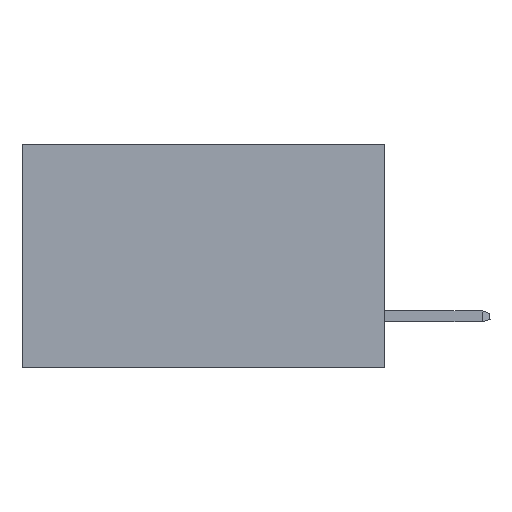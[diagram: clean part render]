
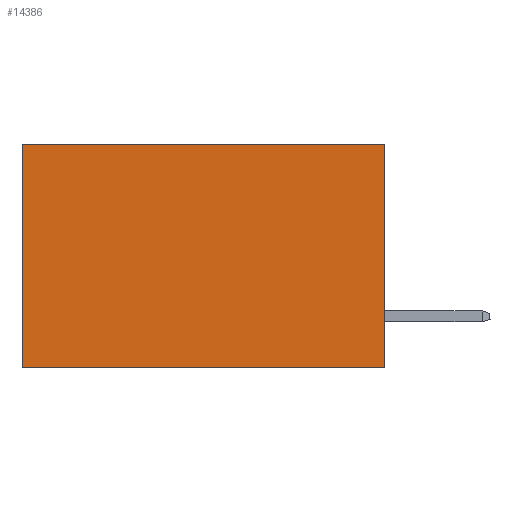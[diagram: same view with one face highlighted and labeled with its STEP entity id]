
A CAD part, left-side view. The second image highlights one B-rep face of the part: STEP entity #14386.
In plain terms, the highlighted planar face has unit normal (-1, 0, 0).
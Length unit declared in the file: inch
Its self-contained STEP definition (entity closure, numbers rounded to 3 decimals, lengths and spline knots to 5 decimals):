
#104 = VECTOR ( 'NONE', #4409, 39.37008 ) ;
#169 = VECTOR ( 'NONE', #10828, 39.37008 ) ;
#344 = ORIENTED_EDGE ( 'NONE', *, *, #9839, .F. ) ;
#633 = DIRECTION ( 'NONE',  ( 0., 0., -1. ) ) ;
#2063 = CARTESIAN_POINT ( 'NONE',  ( 0.298, 0.6, 0. ) ) ;
#2484 = ORIENTED_EDGE ( 'NONE', *, *, #14742, .T. ) ;
#2728 = ORIENTED_EDGE ( 'NONE', *, *, #3739, .F. ) ;
#3150 = CARTESIAN_POINT ( 'NONE',  ( 0.298, 0., 0. ) ) ;
#3463 = CARTESIAN_POINT ( 'NONE',  ( 0.298, 0.6, -0.37 ) ) ;
#3540 = VERTEX_POINT ( 'NONE', #12325 ) ;
#3739 = EDGE_CURVE ( 'NONE', #7100, #16364, #4299, .T. ) ;
#3740 = DIRECTION ( 'NONE',  ( 0., 1., 0. ) ) ;
#3833 = LINE ( 'NONE', #9637, #4688 ) ;
#4299 = LINE ( 'NONE', #13336, #6196 ) ;
#4409 = DIRECTION ( 'NONE',  ( 0., 1., 0. ) ) ;
#4688 = VECTOR ( 'NONE', #13706, 39.37008 ) ;
#6084 = PLANE ( 'NONE',  #12268 ) ;
#6181 = VERTEX_POINT ( 'NONE', #13823 ) ;
#6196 = VECTOR ( 'NONE', #3740, 39.37008 ) ;
#7100 = VERTEX_POINT ( 'NONE', #10840 ) ;
#7273 = LINE ( 'NONE', #3150, #104 ) ;
#8187 = LINE ( 'NONE', #2063, #169 ) ;
#8215 = EDGE_CURVE ( 'NONE', #6181, #3540, #7273, .T. ) ;
#8732 = CARTESIAN_POINT ( 'NONE',  ( 0.298, 0., 0. ) ) ;
#8881 = ORIENTED_EDGE ( 'NONE', *, *, #8215, .T. ) ;
#9637 = CARTESIAN_POINT ( 'NONE',  ( 0.298, 0., 0. ) ) ;
#9839 = EDGE_CURVE ( 'NONE', #6181, #7100, #3833, .T. ) ;
#10828 = DIRECTION ( 'NONE',  ( 0., 0., -1. ) ) ;
#10840 = CARTESIAN_POINT ( 'NONE',  ( 0.298, 0., -0.37 ) ) ;
#11397 = DIRECTION ( 'NONE',  ( 1., 0., 0. ) ) ;
#12268 = AXIS2_PLACEMENT_3D ( 'NONE', #8732, #11397, #633 ) ;
#12325 = CARTESIAN_POINT ( 'NONE',  ( 0.298, 0.6, 0. ) ) ;
#13336 = CARTESIAN_POINT ( 'NONE',  ( 0.298, 0., -0.37 ) ) ;
#13706 = DIRECTION ( 'NONE',  ( 0., 0., -1. ) ) ;
#13823 = CARTESIAN_POINT ( 'NONE',  ( 0.298, 0., 0. ) ) ;
#14386 = ADVANCED_FACE ( 'NONE', ( #16250 ), #6084, .F. ) ;
#14548 = EDGE_LOOP ( 'NONE', ( #2484, #2728, #344, #8881 ) ) ;
#14742 = EDGE_CURVE ( 'NONE', #3540, #16364, #8187, .T. ) ;
#16250 = FACE_OUTER_BOUND ( 'NONE', #14548, .T. ) ;
#16364 = VERTEX_POINT ( 'NONE', #3463 ) ;
